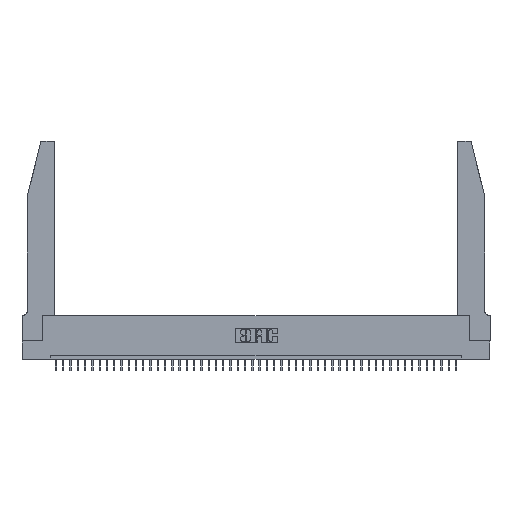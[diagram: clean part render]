
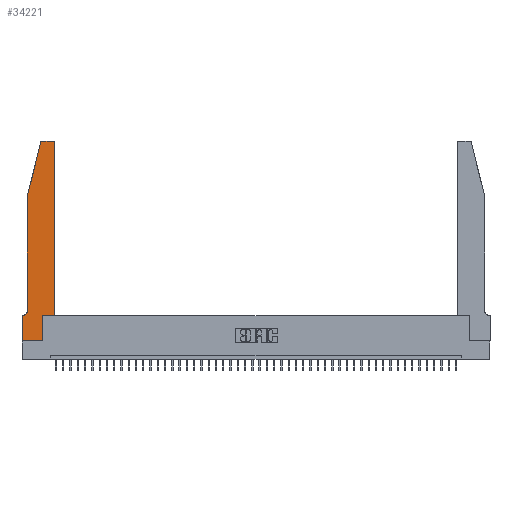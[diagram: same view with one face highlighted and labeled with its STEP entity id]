
A CAD part, top view. The second image highlights one B-rep face of the part: STEP entity #34221.
In plain terms, the highlighted planar face has unit normal (0, 0, 1).
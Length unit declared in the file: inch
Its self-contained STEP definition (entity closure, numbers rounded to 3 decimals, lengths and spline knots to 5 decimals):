
#351 = CARTESIAN_POINT ( 'NONE',  ( 0.25487, 2.72718, 0.37 ) ) ;
#367 = LINE ( 'NONE', #5787, #26535 ) ;
#1293 = CARTESIAN_POINT ( 'NONE',  ( 0.4505, 0.35, 0.37 ) ) ;
#2107 = DIRECTION ( 'NONE',  ( 0., 1., 0. ) ) ;
#2763 = CARTESIAN_POINT ( 'NONE',  ( 0., 0., 0.37 ) ) ;
#2876 = LINE ( 'NONE', #40084, #20301 ) ;
#3958 = LINE ( 'NONE', #7665, #32827 ) ;
#4608 = EDGE_CURVE ( 'NONE', #8934, #30493, #27211, .T. ) ;
#5366 = DIRECTION ( 'NONE',  ( 0., 0., 1. ) ) ;
#5787 = CARTESIAN_POINT ( 'NONE',  ( 0.2865, 0.35, 0.37 ) ) ;
#6138 = ORIENTED_EDGE ( 'NONE', *, *, #8877, .T. ) ;
#7537 = LINE ( 'NONE', #1293, #39060 ) ;
#7586 = VERTEX_POINT ( 'NONE', #44314 ) ;
#7665 = CARTESIAN_POINT ( 'NONE',  ( 0.2605, 2.75, 0.37 ) ) ;
#7819 = PLANE ( 'NONE',  #20127 ) ;
#7950 = DIRECTION ( 'NONE',  ( 1., 0., 0. ) ) ;
#7968 = EDGE_LOOP ( 'NONE', ( #13623, #19472, #32282, #30438, #6138, #30474, #17781, #21666, #18338, #17724, #32811, #14197 ) ) ;
#8554 = VERTEX_POINT ( 'NONE', #351 ) ;
#8675 = EDGE_CURVE ( 'NONE', #10210, #7586, #30161, .T. ) ;
#8697 = CARTESIAN_POINT ( 'NONE',  ( 0.0055, 0.42, 0.37 ) ) ;
#8828 = VERTEX_POINT ( 'NONE', #12519 ) ;
#8877 = EDGE_CURVE ( 'NONE', #26640, #8828, #42101, .T. ) ;
#8934 = VERTEX_POINT ( 'NONE', #2763 ) ;
#10210 = VERTEX_POINT ( 'NONE', #20156 ) ;
#11157 = VERTEX_POINT ( 'NONE', #30844 ) ;
#11208 = CARTESIAN_POINT ( 'NONE',  ( 0.0755, 2., 0.37 ) ) ;
#11509 = CARTESIAN_POINT ( 'NONE',  ( 0.0755, 2., 0.37 ) ) ;
#11806 = CARTESIAN_POINT ( 'NONE',  ( 0.0755, 0.42, 0.37 ) ) ;
#11909 = CARTESIAN_POINT ( 'NONE',  ( 0.284, 2.72, 0.37 ) ) ;
#12068 = DIRECTION ( 'NONE',  ( -1., 0., 0. ) ) ;
#12487 = AXIS2_PLACEMENT_3D ( 'NONE', #11909, #5366, #18906 ) ;
#12519 = CARTESIAN_POINT ( 'NONE',  ( 0.0055, 0.35, 0.37 ) ) ;
#12810 = AXIS2_PLACEMENT_3D ( 'NONE', #8697, #29366, #12068 ) ;
#13623 = ORIENTED_EDGE ( 'NONE', *, *, #21433, .T. ) ;
#13853 = CARTESIAN_POINT ( 'NONE',  ( 0.2865, 0., 0.37 ) ) ;
#14083 = EDGE_CURVE ( 'NONE', #29504, #15046, #7537, .T. ) ;
#14197 = ORIENTED_EDGE ( 'NONE', *, *, #8675, .T. ) ;
#14746 = EDGE_CURVE ( 'NONE', #30493, #29504, #367, .T. ) ;
#15046 = VERTEX_POINT ( 'NONE', #38276 ) ;
#15162 = EDGE_CURVE ( 'NONE', #24898, #26640, #36823, .T. ) ;
#15787 = DIRECTION ( 'NONE',  ( 1., 0., 0. ) ) ;
#16137 = EDGE_CURVE ( 'NONE', #8554, #24898, #35086, .T. ) ;
#17724 = ORIENTED_EDGE ( 'NONE', *, *, #14083, .T. ) ;
#17781 = ORIENTED_EDGE ( 'NONE', *, *, #36944, .T. ) ;
#18174 = DIRECTION ( 'NONE',  ( -1., 0., 0. ) ) ;
#18215 = EDGE_CURVE ( 'NONE', #11157, #8554, #39120, .T. ) ;
#18338 = ORIENTED_EDGE ( 'NONE', *, *, #14746, .T. ) ;
#18906 = DIRECTION ( 'NONE',  ( 1., 0., 0. ) ) ;
#19220 = VECTOR ( 'NONE', #27860, 39.37008 ) ;
#19472 = ORIENTED_EDGE ( 'NONE', *, *, #18215, .T. ) ;
#19575 = VECTOR ( 'NONE', #15787, 39.37008 ) ;
#20127 = AXIS2_PLACEMENT_3D ( 'NONE', #32009, #22157, #25012 ) ;
#20156 = CARTESIAN_POINT ( 'NONE',  ( 0.4505, 2.72, 0.37 ) ) ;
#20301 = VECTOR ( 'NONE', #43896, 39.37008 ) ;
#20667 = VECTOR ( 'NONE', #34022, 39.37008 ) ;
#21227 = CARTESIAN_POINT ( 'NONE',  ( 0.2865, 0.35, 0.37 ) ) ;
#21433 = EDGE_CURVE ( 'NONE', #7586, #11157, #3958, .T. ) ;
#21666 = ORIENTED_EDGE ( 'NONE', *, *, #4608, .T. ) ;
#21720 = DIRECTION ( 'NONE',  ( 1., 0., 0. ) ) ;
#22157 = DIRECTION ( 'NONE',  ( 0., 0., 1. ) ) ;
#22869 = LINE ( 'NONE', #23564, #20667 ) ;
#23564 = CARTESIAN_POINT ( 'NONE',  ( 0.4505, 0.35, 0.37 ) ) ;
#24898 = VERTEX_POINT ( 'NONE', #11208 ) ;
#25012 = DIRECTION ( 'NONE',  ( 1., 0., 0. ) ) ;
#25845 = VECTOR ( 'NONE', #41532, 39.37008 ) ;
#26394 = EDGE_CURVE ( 'NONE', #15046, #10210, #22869, .T. ) ;
#26535 = VECTOR ( 'NONE', #2107, 39.37008 ) ;
#26640 = VERTEX_POINT ( 'NONE', #11806 ) ;
#27056 = VECTOR ( 'NONE', #43121, 39.37008 ) ;
#27211 = LINE ( 'NONE', #36607, #19575 ) ;
#27710 = CARTESIAN_POINT ( 'NONE',  ( 0.0755, 0.35, 0.37 ) ) ;
#27860 = DIRECTION ( 'NONE',  ( -1., 0., 0. ) ) ;
#29366 = DIRECTION ( 'NONE',  ( 0., 0., -1. ) ) ;
#29504 = VERTEX_POINT ( 'NONE', #21227 ) ;
#29972 = AXIS2_PLACEMENT_3D ( 'NONE', #35790, #39260, #7950 ) ;
#30161 = CIRCLE ( 'NONE', #29972, 0.03 ) ;
#30438 = ORIENTED_EDGE ( 'NONE', *, *, #15162, .T. ) ;
#30474 = ORIENTED_EDGE ( 'NONE', *, *, #44988, .T. ) ;
#30493 = VERTEX_POINT ( 'NONE', #13853 ) ;
#30844 = CARTESIAN_POINT ( 'NONE',  ( 0.284, 2.75, 0.37 ) ) ;
#31807 = FACE_OUTER_BOUND ( 'NONE', #7968, .T. ) ;
#32009 = CARTESIAN_POINT ( 'NONE',  ( 0., 0.35, 0.37 ) ) ;
#32282 = ORIENTED_EDGE ( 'NONE', *, *, #16137, .T. ) ;
#32811 = ORIENTED_EDGE ( 'NONE', *, *, #26394, .T. ) ;
#32827 = VECTOR ( 'NONE', #18174, 39.37008 ) ;
#34022 = DIRECTION ( 'NONE',  ( 0., 1., 0. ) ) ;
#34221 = ADVANCED_FACE ( 'NONE', ( #31807 ), #7819, .T. ) ;
#34394 = CARTESIAN_POINT ( 'NONE',  ( 0.0755, 2., 0.37 ) ) ;
#35086 = LINE ( 'NONE', #34394, #25845 ) ;
#35790 = CARTESIAN_POINT ( 'NONE',  ( 0.4205, 2.72, 0.37 ) ) ;
#36607 = CARTESIAN_POINT ( 'NONE',  ( 0., 0., 0.37 ) ) ;
#36823 = LINE ( 'NONE', #11509, #27056 ) ;
#36944 = EDGE_CURVE ( 'NONE', #39758, #8934, #2876, .T. ) ;
#37373 = CARTESIAN_POINT ( 'NONE',  ( 0., 0.35, 0.37 ) ) ;
#38276 = CARTESIAN_POINT ( 'NONE',  ( 0.4505, 0.35, 0.37 ) ) ;
#39060 = VECTOR ( 'NONE', #21720, 39.37008 ) ;
#39120 = CIRCLE ( 'NONE', #12487, 0.03 ) ;
#39260 = DIRECTION ( 'NONE',  ( 0., 0., 1. ) ) ;
#39758 = VERTEX_POINT ( 'NONE', #37373 ) ;
#40084 = CARTESIAN_POINT ( 'NONE',  ( 0., 0., 0.37 ) ) ;
#41532 = DIRECTION ( 'NONE',  ( -0.239, -0.971, 0. ) ) ;
#42101 = CIRCLE ( 'NONE', #12810, 0.07 ) ;
#42532 = LINE ( 'NONE', #27710, #19220 ) ;
#43121 = DIRECTION ( 'NONE',  ( 0., -1., 0. ) ) ;
#43896 = DIRECTION ( 'NONE',  ( 0., -1., 0. ) ) ;
#44314 = CARTESIAN_POINT ( 'NONE',  ( 0.4205, 2.75, 0.37 ) ) ;
#44988 = EDGE_CURVE ( 'NONE', #8828, #39758, #42532, .T. ) ;
